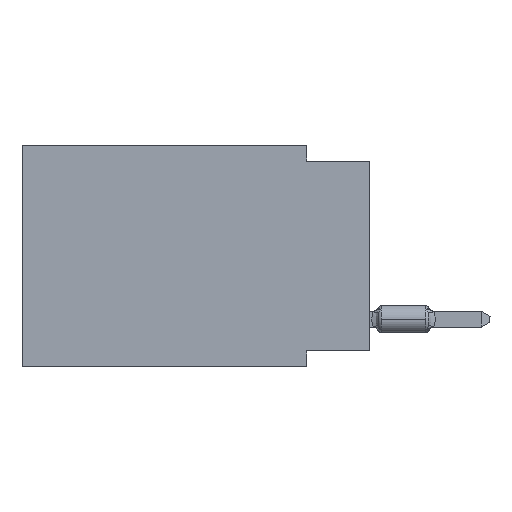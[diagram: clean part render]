
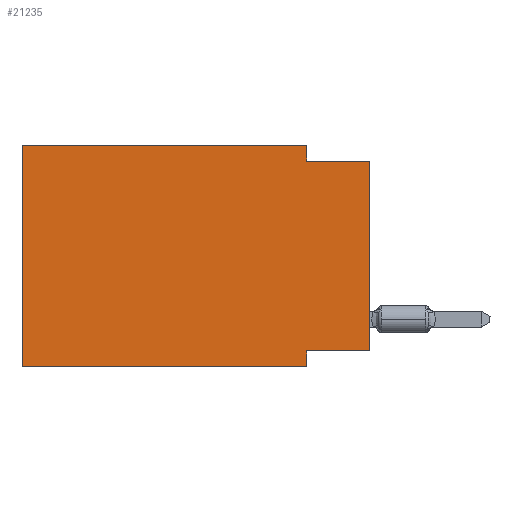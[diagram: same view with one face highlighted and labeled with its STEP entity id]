
A CAD part, left-side view. The second image highlights one B-rep face of the part: STEP entity #21235.
In plain terms, the highlighted planar face has unit normal (-1, 0, 0).
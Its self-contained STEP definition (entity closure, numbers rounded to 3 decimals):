
#778 = DIRECTION ( 'NONE',  ( 0., 0., -1. ) ) ;
#1017 = VERTEX_POINT ( 'NONE', #27225 ) ;
#1210 = CARTESIAN_POINT ( 'NONE',  ( 0., 2.54, 0. ) ) ;
#1892 = CARTESIAN_POINT ( 'NONE',  ( 0., 2.54, -0.635 ) ) ;
#3735 = CARTESIAN_POINT ( 'NONE',  ( 0., 0., -8.255 ) ) ;
#4149 = CARTESIAN_POINT ( 'NONE',  ( 0., 2.54, -8.255 ) ) ;
#4866 = VECTOR ( 'NONE', #44023, 1000. ) ;
#4873 = LINE ( 'NONE', #1210, #48222 ) ;
#5044 = EDGE_CURVE ( 'NONE', #1017, #49218, #24845, .T. ) ;
#5649 = EDGE_CURVE ( 'NONE', #16921, #32336, #50012, .T. ) ;
#8294 = DIRECTION ( 'NONE',  ( 0., 0., 1. ) ) ;
#9746 = DIRECTION ( 'NONE',  ( 0., 1., 0. ) ) ;
#11261 = VECTOR ( 'NONE', #47071, 1000. ) ;
#13134 = DIRECTION ( 'NONE',  ( 0., -1., 0. ) ) ;
#13378 = DIRECTION ( 'NONE',  ( 0., -1., 0. ) ) ;
#13682 = CARTESIAN_POINT ( 'NONE',  ( 0., 13.97, -8.89 ) ) ;
#14318 = LINE ( 'NONE', #32905, #53648 ) ;
#15154 = ORIENTED_EDGE ( 'NONE', *, *, #55939, .F. ) ;
#16889 = CARTESIAN_POINT ( 'NONE',  ( 0., 0., -0.635 ) ) ;
#16921 = VERTEX_POINT ( 'NONE', #3735 ) ;
#18391 = ORIENTED_EDGE ( 'NONE', *, *, #29110, .T. ) ;
#18428 = DIRECTION ( 'NONE',  ( 1., 0., 0. ) ) ;
#19180 = DIRECTION ( 'NONE',  ( 0., 0., -1. ) ) ;
#20229 = VECTOR ( 'NONE', #13378, 1000. ) ;
#21235 = ADVANCED_FACE ( 'NONE', ( #23890 ), #42507, .F. ) ;
#23890 = FACE_OUTER_BOUND ( 'NONE', #43062, .T. ) ;
#24845 = LINE ( 'NONE', #57167, #4866 ) ;
#27225 = CARTESIAN_POINT ( 'NONE',  ( 0., 13.97, -8.89 ) ) ;
#27453 = EDGE_CURVE ( 'NONE', #40992, #32336, #36297, .T. ) ;
#27747 = CARTESIAN_POINT ( 'NONE',  ( 0., 2.54, -8.89 ) ) ;
#29110 = EDGE_CURVE ( 'NONE', #1017, #51037, #32267, .T. ) ;
#29442 = ORIENTED_EDGE ( 'NONE', *, *, #27453, .F. ) ;
#32267 = LINE ( 'NONE', #13682, #20229 ) ;
#32336 = VERTEX_POINT ( 'NONE', #16889 ) ;
#32382 = ORIENTED_EDGE ( 'NONE', *, *, #5044, .F. ) ;
#32905 = CARTESIAN_POINT ( 'NONE',  ( 0., 0., -8.255 ) ) ;
#34578 = VERTEX_POINT ( 'NONE', #45658 ) ;
#35408 = CARTESIAN_POINT ( 'NONE',  ( 0., 0., 0. ) ) ;
#36297 = LINE ( 'NONE', #50902, #47364 ) ;
#40011 = VECTOR ( 'NONE', #46346, 1000. ) ;
#40648 = CARTESIAN_POINT ( 'NONE',  ( 0., 13.97, 0. ) ) ;
#40992 = VERTEX_POINT ( 'NONE', #1892 ) ;
#41628 = CARTESIAN_POINT ( 'NONE',  ( 0., 13.97, 0. ) ) ;
#42217 = LINE ( 'NONE', #41628, #11261 ) ;
#42507 = PLANE ( 'NONE',  #47369 ) ;
#42844 = EDGE_CURVE ( 'NONE', #34578, #40992, #4873, .T. ) ;
#43062 = EDGE_LOOP ( 'NONE', ( #43667, #29442, #47308, #54672, #32382, #18391, #15154, #49115 ) ) ;
#43667 = ORIENTED_EDGE ( 'NONE', *, *, #5649, .T. ) ;
#44023 = DIRECTION ( 'NONE',  ( 0., 0., 1. ) ) ;
#45658 = CARTESIAN_POINT ( 'NONE',  ( 0., 2.54, 0. ) ) ;
#46346 = DIRECTION ( 'NONE',  ( 0., 0., -1. ) ) ;
#47071 = DIRECTION ( 'NONE',  ( 0., -1., 0. ) ) ;
#47308 = ORIENTED_EDGE ( 'NONE', *, *, #42844, .F. ) ;
#47364 = VECTOR ( 'NONE', #13134, 1000. ) ;
#47369 = AXIS2_PLACEMENT_3D ( 'NONE', #51021, #18428, #778 ) ;
#48222 = VECTOR ( 'NONE', #19180, 1000. ) ;
#48939 = EDGE_CURVE ( 'NONE', #49218, #34578, #42217, .T. ) ;
#49115 = ORIENTED_EDGE ( 'NONE', *, *, #56190, .F. ) ;
#49218 = VERTEX_POINT ( 'NONE', #40648 ) ;
#50012 = LINE ( 'NONE', #35408, #55330 ) ;
#50901 = LINE ( 'NONE', #27747, #40011 ) ;
#50902 = CARTESIAN_POINT ( 'NONE',  ( 0., 0., -0.635 ) ) ;
#51021 = CARTESIAN_POINT ( 'NONE',  ( 0., 13.97, 0. ) ) ;
#51037 = VERTEX_POINT ( 'NONE', #55498 ) ;
#53648 = VECTOR ( 'NONE', #9746, 1000. ) ;
#54672 = ORIENTED_EDGE ( 'NONE', *, *, #48939, .F. ) ;
#55330 = VECTOR ( 'NONE', #8294, 1000. ) ;
#55498 = CARTESIAN_POINT ( 'NONE',  ( 0., 2.54, -8.89 ) ) ;
#55939 = EDGE_CURVE ( 'NONE', #60201, #51037, #50901, .T. ) ;
#56190 = EDGE_CURVE ( 'NONE', #16921, #60201, #14318, .T. ) ;
#57167 = CARTESIAN_POINT ( 'NONE',  ( 0., 13.97, 0. ) ) ;
#60201 = VERTEX_POINT ( 'NONE', #4149 ) ;
